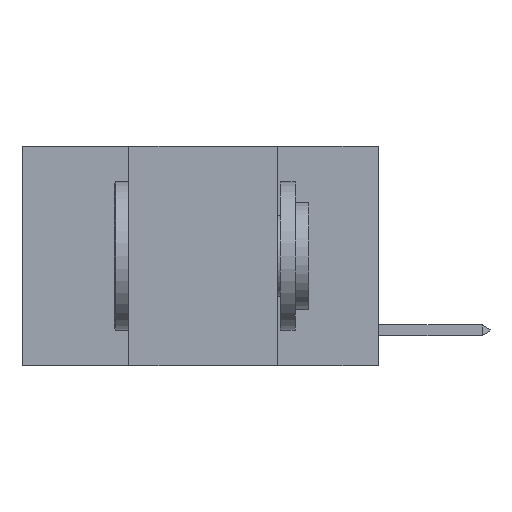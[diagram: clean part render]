
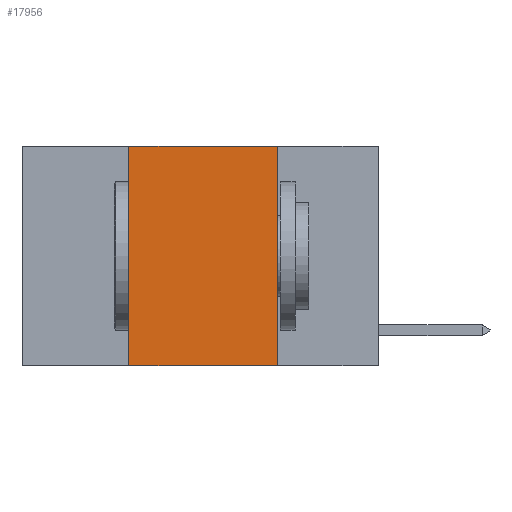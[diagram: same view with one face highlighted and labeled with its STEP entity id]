
A CAD part, left-side view. The second image highlights one B-rep face of the part: STEP entity #17956.
In plain terms, the highlighted planar face has unit normal (-1, 0, 0).
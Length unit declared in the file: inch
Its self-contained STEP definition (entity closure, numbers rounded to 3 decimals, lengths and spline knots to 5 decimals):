
#44 = VECTOR ( 'NONE', #11141, 39.37008 ) ;
#108 = PLANE ( 'NONE',  #5135 ) ;
#366 = VERTEX_POINT ( 'NONE', #12765 ) ;
#481 = FACE_OUTER_BOUND ( 'NONE', #5239, .T. ) ;
#724 = CARTESIAN_POINT ( 'NONE',  ( 0., 0.42, -0.37 ) ) ;
#1001 = VERTEX_POINT ( 'NONE', #724 ) ;
#3064 = DIRECTION ( 'NONE',  ( 0., 0., -1. ) ) ;
#3566 = LINE ( 'NONE', #13552, #12897 ) ;
#3595 = EDGE_CURVE ( 'NONE', #366, #12933, #14620, .T. ) ;
#4114 = CARTESIAN_POINT ( 'NONE',  ( 0., 0.17, -0.37 ) ) ;
#5135 = AXIS2_PLACEMENT_3D ( 'NONE', #10146, #10235, #3064 ) ;
#5239 = EDGE_LOOP ( 'NONE', ( #7567, #15763, #12352, #7759 ) ) ;
#5663 = CARTESIAN_POINT ( 'NONE',  ( 0., 0.42, 0. ) ) ;
#6567 = LINE ( 'NONE', #9969, #44 ) ;
#7567 = ORIENTED_EDGE ( 'NONE', *, *, #13586, .F. ) ;
#7659 = DIRECTION ( 'NONE',  ( 0., -1., 0. ) ) ;
#7759 = ORIENTED_EDGE ( 'NONE', *, *, #10857, .T. ) ;
#7790 = DIRECTION ( 'NONE',  ( 0., 0., -1. ) ) ;
#8931 = CARTESIAN_POINT ( 'NONE',  ( 0., 0.17, 0. ) ) ;
#8955 = CARTESIAN_POINT ( 'NONE',  ( 0., 0.6, 0. ) ) ;
#9717 = LINE ( 'NONE', #5663, #15433 ) ;
#9969 = CARTESIAN_POINT ( 'NONE',  ( 0., 0.6, -0.37 ) ) ;
#10146 = CARTESIAN_POINT ( 'NONE',  ( 0., 0.6, 0. ) ) ;
#10235 = DIRECTION ( 'NONE',  ( 1., 0., 0. ) ) ;
#10407 = EDGE_CURVE ( 'NONE', #1001, #366, #9717, .T. ) ;
#10857 = EDGE_CURVE ( 'NONE', #1001, #13707, #6567, .T. ) ;
#11141 = DIRECTION ( 'NONE',  ( 0., -1., 0. ) ) ;
#12352 = ORIENTED_EDGE ( 'NONE', *, *, #10407, .F. ) ;
#12765 = CARTESIAN_POINT ( 'NONE',  ( 0., 0.42, 0. ) ) ;
#12787 = DIRECTION ( 'NONE',  ( 0., 0., 1. ) ) ;
#12897 = VECTOR ( 'NONE', #7790, 39.37008 ) ;
#12933 = VERTEX_POINT ( 'NONE', #8931 ) ;
#13327 = VECTOR ( 'NONE', #7659, 39.37008 ) ;
#13552 = CARTESIAN_POINT ( 'NONE',  ( 0., 0.17, 0. ) ) ;
#13586 = EDGE_CURVE ( 'NONE', #12933, #13707, #3566, .T. ) ;
#13707 = VERTEX_POINT ( 'NONE', #4114 ) ;
#14620 = LINE ( 'NONE', #8955, #13327 ) ;
#15433 = VECTOR ( 'NONE', #12787, 39.37008 ) ;
#15763 = ORIENTED_EDGE ( 'NONE', *, *, #3595, .F. ) ;
#17956 = ADVANCED_FACE ( 'NONE', ( #481 ), #108, .F. ) ;
